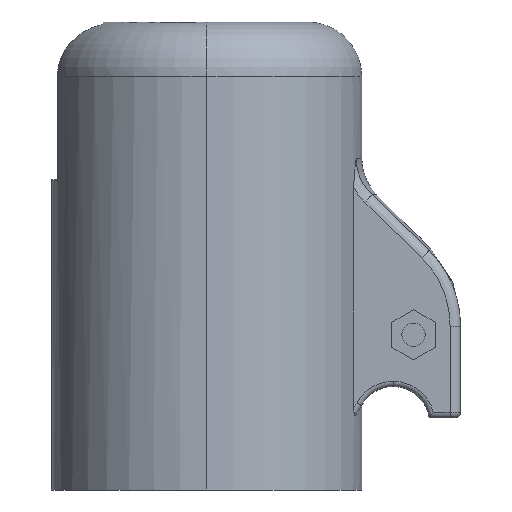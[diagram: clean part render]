
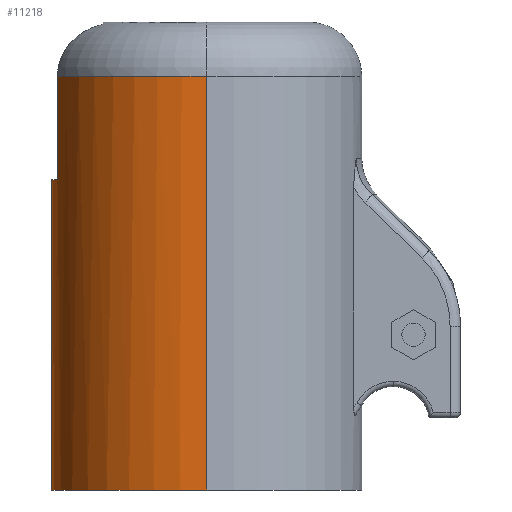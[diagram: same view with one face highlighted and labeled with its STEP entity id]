
A CAD part, left-side view. The second image highlights one B-rep face of the part: STEP entity #11218.
In plain terms, the highlighted cylindrical face has radius 15 mm (diameter 30 mm), a partial arc.
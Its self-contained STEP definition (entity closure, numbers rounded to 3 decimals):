
#30 = DIRECTION ( 'NONE',  ( 0., 0., -1. ) ) ;
#746 = ORIENTED_EDGE ( 'NONE', *, *, #14635, .T. ) ;
#1358 = EDGE_CURVE ( 'NONE', #1950, #13795, #11397, .T. ) ;
#1620 = CARTESIAN_POINT ( 'NONE',  ( 15., 0., 40. ) ) ;
#1720 = LINE ( 'NONE', #2423, #9162 ) ;
#1785 = CARTESIAN_POINT ( 'NONE',  ( 0., 0., 40. ) ) ;
#1950 = VERTEX_POINT ( 'NONE', #10426 ) ;
#2423 = CARTESIAN_POINT ( 'NONE',  ( -4.115, 14.424, 30. ) ) ;
#2655 = VERTEX_POINT ( 'NONE', #13420 ) ;
#2833 = AXIS2_PLACEMENT_3D ( 'NONE', #1785, #12180, #3265 ) ;
#2848 = EDGE_CURVE ( 'NONE', #13795, #6658, #10894, .T. ) ;
#3019 = CARTESIAN_POINT ( 'NONE',  ( 0., 0., 0. ) ) ;
#3062 = DIRECTION ( 'NONE',  ( 0., 0., -1. ) ) ;
#3265 = DIRECTION ( 'NONE',  ( 1., 0., 0. ) ) ;
#3434 = CIRCLE ( 'NONE', #5720, 15. ) ;
#3577 = CARTESIAN_POINT ( 'NONE',  ( 4.115, 14.424, 30. ) ) ;
#4064 = DIRECTION ( 'NONE',  ( -1., 0., 0. ) ) ;
#4071 = CARTESIAN_POINT ( 'NONE',  ( 15., 0., 40. ) ) ;
#4117 = EDGE_CURVE ( 'NONE', #6658, #13571, #4810, .T. ) ;
#4523 = DIRECTION ( 'NONE',  ( 1., 0., 0. ) ) ;
#4670 = ORIENTED_EDGE ( 'NONE', *, *, #1358, .T. ) ;
#4810 = CIRCLE ( 'NONE', #4860, 15. ) ;
#4860 = AXIS2_PLACEMENT_3D ( 'NONE', #3019, #13423, #4523 ) ;
#5375 = EDGE_CURVE ( 'NONE', #2655, #13571, #6666, .T. ) ;
#5720 = AXIS2_PLACEMENT_3D ( 'NONE', #8962, #30, #10477 ) ;
#6255 = DIRECTION ( 'NONE',  ( 0., 0., 1. ) ) ;
#6658 = VERTEX_POINT ( 'NONE', #10669 ) ;
#6666 = LINE ( 'NONE', #14112, #9708 ) ;
#6762 = CIRCLE ( 'NONE', #15831, 15. ) ;
#7914 = ORIENTED_EDGE ( 'NONE', *, *, #12483, .T. ) ;
#7977 = DIRECTION ( 'NONE',  ( 0., 0., -1. ) ) ;
#7997 = ORIENTED_EDGE ( 'NONE', *, *, #5375, .F. ) ;
#8821 = CARTESIAN_POINT ( 'NONE',  ( -4.115, 14.424, 40. ) ) ;
#8895 = ORIENTED_EDGE ( 'NONE', *, *, #10017, .F. ) ;
#8899 = ORIENTED_EDGE ( 'NONE', *, *, #11257, .F. ) ;
#8962 = CARTESIAN_POINT ( 'NONE',  ( 0., 0., 40. ) ) ;
#9162 = VECTOR ( 'NONE', #17334, 1000. ) ;
#9619 = ORIENTED_EDGE ( 'NONE', *, *, #4117, .T. ) ;
#9708 = VECTOR ( 'NONE', #14236, 1000. ) ;
#10017 = EDGE_CURVE ( 'NONE', #18721, #10552, #1720, .T. ) ;
#10279 = CYLINDRICAL_SURFACE ( 'NONE', #18830, 15. ) ;
#10426 = CARTESIAN_POINT ( 'NONE',  ( 4.115, 14.424, 40. ) ) ;
#10444 = VECTOR ( 'NONE', #7977, 1000. ) ;
#10477 = DIRECTION ( 'NONE',  ( 1., 0., 0. ) ) ;
#10552 = VERTEX_POINT ( 'NONE', #8821 ) ;
#10669 = CARTESIAN_POINT ( 'NONE',  ( 15., 0., 0. ) ) ;
#10894 = LINE ( 'NONE', #1620, #10444 ) ;
#11218 = ADVANCED_FACE ( 'NONE', ( #14168 ), #10279, .T. ) ;
#11257 = EDGE_CURVE ( 'NONE', #14963, #18721, #6762, .T. ) ;
#11397 = CIRCLE ( 'NONE', #2833, 15. ) ;
#11642 = LINE ( 'NONE', #14453, #12083 ) ;
#11982 = CARTESIAN_POINT ( 'NONE',  ( 0., 0., 40. ) ) ;
#12083 = VECTOR ( 'NONE', #16054, 1000. ) ;
#12180 = DIRECTION ( 'NONE',  ( 0., 0., -1. ) ) ;
#12483 = EDGE_CURVE ( 'NONE', #14963, #1950, #11642, .T. ) ;
#13420 = CARTESIAN_POINT ( 'NONE',  ( -15., 0., 40. ) ) ;
#13423 = DIRECTION ( 'NONE',  ( 0., 0., 1. ) ) ;
#13491 = CARTESIAN_POINT ( 'NONE',  ( -15., 0., 0. ) ) ;
#13571 = VERTEX_POINT ( 'NONE', #13491 ) ;
#13795 = VERTEX_POINT ( 'NONE', #4071 ) ;
#14112 = CARTESIAN_POINT ( 'NONE',  ( -15., 0., 40. ) ) ;
#14168 = FACE_OUTER_BOUND ( 'NONE', #15042, .T. ) ;
#14236 = DIRECTION ( 'NONE',  ( 0., 0., -1. ) ) ;
#14453 = CARTESIAN_POINT ( 'NONE',  ( 4.115, 14.424, 30. ) ) ;
#14635 = EDGE_CURVE ( 'NONE', #2655, #10552, #3434, .T. ) ;
#14963 = VERTEX_POINT ( 'NONE', #3577 ) ;
#15042 = EDGE_LOOP ( 'NONE', ( #4670, #19217, #9619, #7997, #746, #8895, #8899, #7914 ) ) ;
#15112 = CARTESIAN_POINT ( 'NONE',  ( 0., 0., 30. ) ) ;
#15831 = AXIS2_PLACEMENT_3D ( 'NONE', #15112, #6255, #16610 ) ;
#16054 = DIRECTION ( 'NONE',  ( 0., 0., 1. ) ) ;
#16610 = DIRECTION ( 'NONE',  ( 1., 0., 0. ) ) ;
#17334 = DIRECTION ( 'NONE',  ( 0., 0., 1. ) ) ;
#18182 = CARTESIAN_POINT ( 'NONE',  ( -4.115, 14.424, 30. ) ) ;
#18721 = VERTEX_POINT ( 'NONE', #18182 ) ;
#18830 = AXIS2_PLACEMENT_3D ( 'NONE', #11982, #3062, #4064 ) ;
#19217 = ORIENTED_EDGE ( 'NONE', *, *, #2848, .T. ) ;
